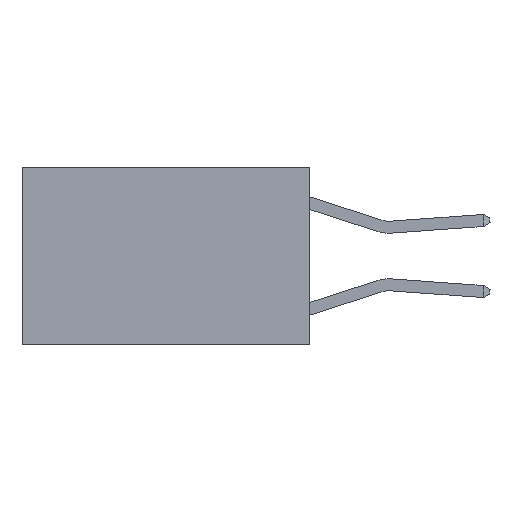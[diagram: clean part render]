
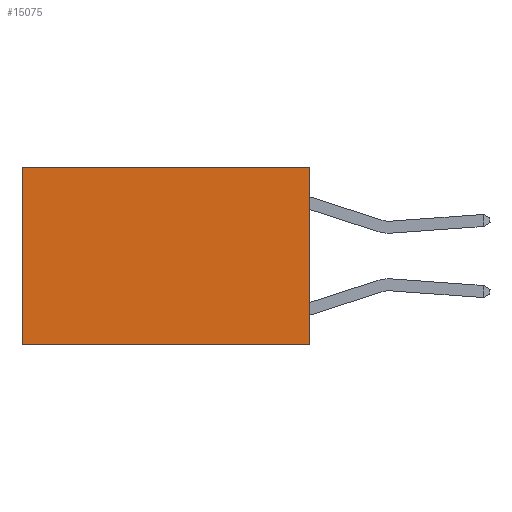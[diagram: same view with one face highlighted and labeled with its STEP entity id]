
A CAD part, left-side view. The second image highlights one B-rep face of the part: STEP entity #15075.
In plain terms, the highlighted planar face has unit normal (-1, 0, 0).
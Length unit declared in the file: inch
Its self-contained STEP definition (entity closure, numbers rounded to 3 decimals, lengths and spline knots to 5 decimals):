
#782 = VERTEX_POINT ( 'NONE', #13721 ) ;
#819 = VECTOR ( 'NONE', #12763, 39.37008 ) ;
#950 = DIRECTION ( 'NONE',  ( 0., 1., 0. ) ) ;
#2194 = EDGE_CURVE ( 'NONE', #3377, #16057, #5632, .T. ) ;
#2550 = VECTOR ( 'NONE', #17097, 39.37008 ) ;
#2974 = CARTESIAN_POINT ( 'NONE',  ( 0.2625, 0.6, 0. ) ) ;
#3377 = VERTEX_POINT ( 'NONE', #7841 ) ;
#3393 = LINE ( 'NONE', #5164, #819 ) ;
#3758 = DIRECTION ( 'NONE',  ( 0., 0., -1. ) ) ;
#5164 = CARTESIAN_POINT ( 'NONE',  ( 0.2625, 0., 0. ) ) ;
#5632 = LINE ( 'NONE', #17914, #11658 ) ;
#6476 = VECTOR ( 'NONE', #18023, 39.37008 ) ;
#6870 = CARTESIAN_POINT ( 'NONE',  ( 0.2625, 0., 0. ) ) ;
#7011 = EDGE_CURVE ( 'NONE', #782, #3377, #16350, .T. ) ;
#7098 = ORIENTED_EDGE ( 'NONE', *, *, #14161, .T. ) ;
#7841 = CARTESIAN_POINT ( 'NONE',  ( 0.2625, 0., -0.37 ) ) ;
#8278 = ORIENTED_EDGE ( 'NONE', *, *, #7011, .F. ) ;
#10120 = FACE_OUTER_BOUND ( 'NONE', #11861, .T. ) ;
#10730 = ORIENTED_EDGE ( 'NONE', *, *, #15661, .T. ) ;
#11478 = PLANE ( 'NONE',  #12490 ) ;
#11658 = VECTOR ( 'NONE', #950, 39.37008 ) ;
#11861 = EDGE_LOOP ( 'NONE', ( #10730, #19652, #8278, #7098 ) ) ;
#12490 = AXIS2_PLACEMENT_3D ( 'NONE', #6870, #14784, #3758 ) ;
#12533 = LINE ( 'NONE', #2974, #2550 ) ;
#12763 = DIRECTION ( 'NONE',  ( 0., 1., 0. ) ) ;
#13721 = CARTESIAN_POINT ( 'NONE',  ( 0.2625, 0., 0. ) ) ;
#14161 = EDGE_CURVE ( 'NONE', #782, #18209, #3393, .T. ) ;
#14784 = DIRECTION ( 'NONE',  ( 1., 0., 0. ) ) ;
#14803 = CARTESIAN_POINT ( 'NONE',  ( 0.2625, 0., 0. ) ) ;
#15075 = ADVANCED_FACE ( 'NONE', ( #10120 ), #11478, .F. ) ;
#15661 = EDGE_CURVE ( 'NONE', #18209, #16057, #12533, .T. ) ;
#16057 = VERTEX_POINT ( 'NONE', #18850 ) ;
#16350 = LINE ( 'NONE', #14803, #6476 ) ;
#17097 = DIRECTION ( 'NONE',  ( 0., 0., -1. ) ) ;
#17914 = CARTESIAN_POINT ( 'NONE',  ( 0.2625, 0., -0.37 ) ) ;
#18023 = DIRECTION ( 'NONE',  ( 0., 0., -1. ) ) ;
#18209 = VERTEX_POINT ( 'NONE', #19639 ) ;
#18850 = CARTESIAN_POINT ( 'NONE',  ( 0.2625, 0.6, -0.37 ) ) ;
#19639 = CARTESIAN_POINT ( 'NONE',  ( 0.2625, 0.6, 0. ) ) ;
#19652 = ORIENTED_EDGE ( 'NONE', *, *, #2194, .F. ) ;
